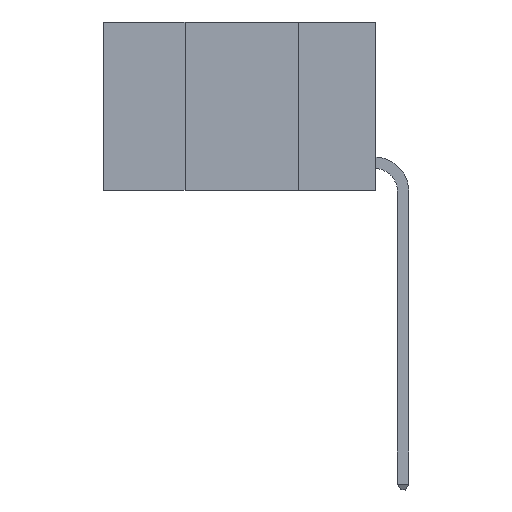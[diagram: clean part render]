
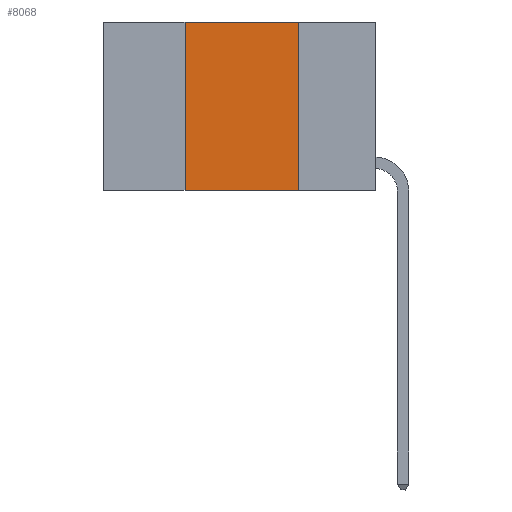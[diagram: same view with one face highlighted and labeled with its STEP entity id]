
A CAD part, left-side view. The second image highlights one B-rep face of the part: STEP entity #8068.
In plain terms, the highlighted planar face has unit normal (-1, 0, 0).
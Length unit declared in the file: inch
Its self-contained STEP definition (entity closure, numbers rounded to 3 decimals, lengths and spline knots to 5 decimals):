
#221 = EDGE_CURVE ( 'NONE', #7058, #8931, #3776, .T. ) ;
#476 = CARTESIAN_POINT ( 'NONE',  ( 0., 0.17, 0. ) ) ;
#486 = EDGE_CURVE ( 'NONE', #6086, #10997, #10589, .T. ) ;
#509 = EDGE_CURVE ( 'NONE', #6086, #8931, #936, .T. ) ;
#936 = LINE ( 'NONE', #11271, #7689 ) ;
#1363 = VECTOR ( 'NONE', #4338, 39.37008 ) ;
#2362 = PLANE ( 'NONE',  #7465 ) ;
#3354 = VECTOR ( 'NONE', #8212, 39.37008 ) ;
#3465 = FACE_OUTER_BOUND ( 'NONE', #9725, .T. ) ;
#3530 = CARTESIAN_POINT ( 'NONE',  ( 0., 0.6, 0. ) ) ;
#3776 = LINE ( 'NONE', #10562, #1363 ) ;
#4138 = DIRECTION ( 'NONE',  ( 1., 0., 0. ) ) ;
#4224 = ORIENTED_EDGE ( 'NONE', *, *, #486, .F. ) ;
#4338 = DIRECTION ( 'NONE',  ( 0., 0., -1. ) ) ;
#4985 = CARTESIAN_POINT ( 'NONE',  ( 0., 0.17, -0.37 ) ) ;
#5042 = LINE ( 'NONE', #3530, #8165 ) ;
#5449 = CARTESIAN_POINT ( 'NONE',  ( 0., 0.42, 0. ) ) ;
#5503 = CARTESIAN_POINT ( 'NONE',  ( 0., 0.42, 0. ) ) ;
#6086 = VERTEX_POINT ( 'NONE', #6339 ) ;
#6339 = CARTESIAN_POINT ( 'NONE',  ( 0., 0.42, -0.37 ) ) ;
#6719 = EDGE_CURVE ( 'NONE', #10997, #7058, #5042, .T. ) ;
#7058 = VERTEX_POINT ( 'NONE', #476 ) ;
#7465 = AXIS2_PLACEMENT_3D ( 'NONE', #9658, #4138, #10524 ) ;
#7689 = VECTOR ( 'NONE', #8200, 39.37008 ) ;
#8068 = ADVANCED_FACE ( 'NONE', ( #3465 ), #2362, .F. ) ;
#8153 = DIRECTION ( 'NONE',  ( 0., -1., 0. ) ) ;
#8165 = VECTOR ( 'NONE', #8153, 39.37008 ) ;
#8200 = DIRECTION ( 'NONE',  ( 0., -1., 0. ) ) ;
#8212 = DIRECTION ( 'NONE',  ( 0., 0., 1. ) ) ;
#8931 = VERTEX_POINT ( 'NONE', #4985 ) ;
#9658 = CARTESIAN_POINT ( 'NONE',  ( 0., 0.6, 0. ) ) ;
#9725 = EDGE_LOOP ( 'NONE', ( #10305, #10252, #4224, #10047 ) ) ;
#10047 = ORIENTED_EDGE ( 'NONE', *, *, #509, .T. ) ;
#10252 = ORIENTED_EDGE ( 'NONE', *, *, #6719, .F. ) ;
#10305 = ORIENTED_EDGE ( 'NONE', *, *, #221, .F. ) ;
#10524 = DIRECTION ( 'NONE',  ( 0., 0., -1. ) ) ;
#10562 = CARTESIAN_POINT ( 'NONE',  ( 0., 0.17, 0. ) ) ;
#10589 = LINE ( 'NONE', #5449, #3354 ) ;
#10997 = VERTEX_POINT ( 'NONE', #5503 ) ;
#11271 = CARTESIAN_POINT ( 'NONE',  ( 0., 0.6, -0.37 ) ) ;
